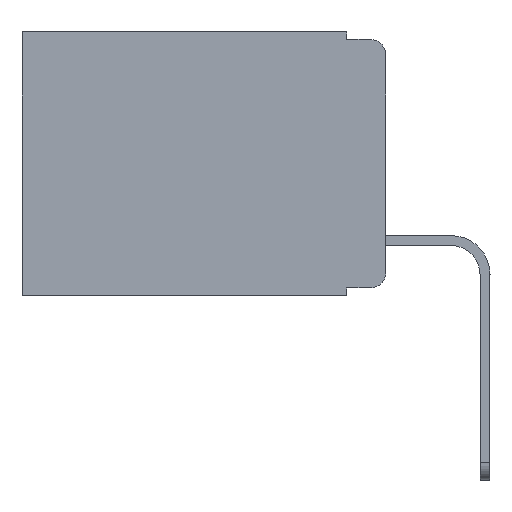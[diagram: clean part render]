
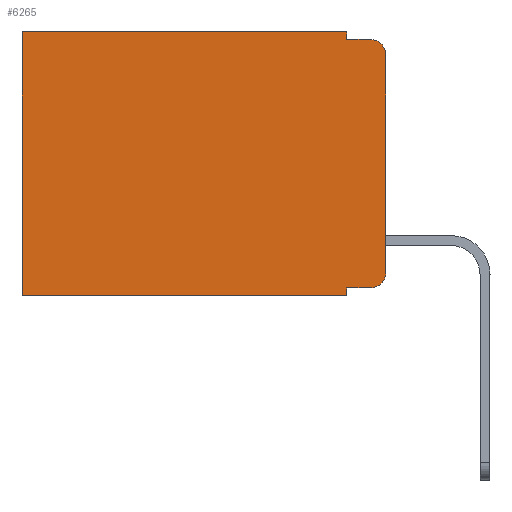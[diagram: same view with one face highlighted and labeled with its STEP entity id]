
A CAD part, left-side view. The second image highlights one B-rep face of the part: STEP entity #6265.
In plain terms, the highlighted planar face has unit normal (-1, 0, 0).
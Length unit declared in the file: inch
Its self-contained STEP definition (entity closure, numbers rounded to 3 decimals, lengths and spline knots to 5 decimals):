
#1 = DIRECTION ( 'NONE',  ( -1., 0., 0. ) ) ;
#213 = CARTESIAN_POINT ( 'NONE',  ( 0.298, 0.051, 0. ) ) ;
#232 = VECTOR ( 'NONE', #8245, 39.37008 ) ;
#307 = CARTESIAN_POINT ( 'NONE',  ( 0.298, 0., -0.03 ) ) ;
#377 = VERTEX_POINT ( 'NONE', #1714 ) ;
#384 = EDGE_CURVE ( 'NONE', #2175, #824, #5941, .T. ) ;
#426 = VERTEX_POINT ( 'NONE', #5489 ) ;
#437 = CARTESIAN_POINT ( 'NONE',  ( 0.298, 0.051, 0. ) ) ;
#585 = DIRECTION ( 'NONE',  ( 0., 1., 0. ) ) ;
#596 = VERTEX_POINT ( 'NONE', #2726 ) ;
#695 = DIRECTION ( 'NONE',  ( 0., 1., 0. ) ) ;
#696 = EDGE_CURVE ( 'NONE', #6378, #426, #6976, .T. ) ;
#824 = VERTEX_POINT ( 'NONE', #2479 ) ;
#828 = LINE ( 'NONE', #5169, #4038 ) ;
#860 = DIRECTION ( 'NONE',  ( 0., 0., -1. ) ) ;
#998 = ORIENTED_EDGE ( 'NONE', *, *, #384, .F. ) ;
#1063 = VECTOR ( 'NONE', #8640, 39.37008 ) ;
#1069 = VERTEX_POINT ( 'NONE', #3045 ) ;
#1148 = ORIENTED_EDGE ( 'NONE', *, *, #696, .T. ) ;
#1170 = AXIS2_PLACEMENT_3D ( 'NONE', #6147, #3266, #1771 ) ;
#1253 = CARTESIAN_POINT ( 'NONE',  ( 0.298, 0.051, -0.333 ) ) ;
#1263 = AXIS2_PLACEMENT_3D ( 'NONE', #8110, #8171, #3757 ) ;
#1367 = CARTESIAN_POINT ( 'NONE',  ( 0.298, 0.02, -0.313 ) ) ;
#1391 = LINE ( 'NONE', #1253, #1063 ) ;
#1530 = EDGE_CURVE ( 'NONE', #824, #426, #4204, .T. ) ;
#1714 = CARTESIAN_POINT ( 'NONE',  ( 0.298, 0.02, -0.333 ) ) ;
#1771 = DIRECTION ( 'NONE',  ( 0., 0., -1. ) ) ;
#1998 = CIRCLE ( 'NONE', #8696, 0.02 ) ;
#2051 = EDGE_CURVE ( 'NONE', #3313, #1069, #7268, .T. ) ;
#2175 = VERTEX_POINT ( 'NONE', #5159 ) ;
#2244 = VECTOR ( 'NONE', #6953, 39.37008 ) ;
#2419 = FACE_OUTER_BOUND ( 'NONE', #6811, .T. ) ;
#2479 = CARTESIAN_POINT ( 'NONE',  ( 0.298, 0.051, -0.01 ) ) ;
#2575 = VECTOR ( 'NONE', #695, 39.37008 ) ;
#2726 = CARTESIAN_POINT ( 'NONE',  ( 0.298, 0., -0.313 ) ) ;
#3045 = CARTESIAN_POINT ( 'NONE',  ( 0.298, 0.473, -0.343 ) ) ;
#3234 = ORIENTED_EDGE ( 'NONE', *, *, #6607, .T. ) ;
#3266 = DIRECTION ( 'NONE',  ( -1., 0., 0. ) ) ;
#3313 = VERTEX_POINT ( 'NONE', #9242 ) ;
#3611 = DIRECTION ( 'NONE',  ( 0., 0., -1. ) ) ;
#3685 = LINE ( 'NONE', #6192, #8020 ) ;
#3757 = DIRECTION ( 'NONE',  ( 0., 0., -1. ) ) ;
#3792 = ORIENTED_EDGE ( 'NONE', *, *, #1530, .F. ) ;
#4014 = CARTESIAN_POINT ( 'NONE',  ( 0.298, 0.051, -0.333 ) ) ;
#4038 = VECTOR ( 'NONE', #860, 39.37008 ) ;
#4204 = LINE ( 'NONE', #4382, #4769 ) ;
#4310 = CARTESIAN_POINT ( 'NONE',  ( 0.298, 0., -0.343 ) ) ;
#4382 = CARTESIAN_POINT ( 'NONE',  ( 0.298, 0.051, -0.01 ) ) ;
#4627 = LINE ( 'NONE', #5634, #8373 ) ;
#4717 = EDGE_CURVE ( 'NONE', #2175, #7197, #4627, .T. ) ;
#4769 = VECTOR ( 'NONE', #8810, 39.37008 ) ;
#4788 = DIRECTION ( 'NONE',  ( 0., 0., -1. ) ) ;
#4868 = EDGE_CURVE ( 'NONE', #377, #596, #1998, .T. ) ;
#4895 = LINE ( 'NONE', #437, #2244 ) ;
#5151 = ORIENTED_EDGE ( 'NONE', *, *, #5830, .T. ) ;
#5159 = CARTESIAN_POINT ( 'NONE',  ( 0.298, 0.051, 0. ) ) ;
#5169 = CARTESIAN_POINT ( 'NONE',  ( 0.298, 0., 0. ) ) ;
#5489 = CARTESIAN_POINT ( 'NONE',  ( 0.298, 0.02, -0.01 ) ) ;
#5634 = CARTESIAN_POINT ( 'NONE',  ( 0.298, 0., 0. ) ) ;
#5711 = EDGE_CURVE ( 'NONE', #6378, #596, #828, .T. ) ;
#5830 = EDGE_CURVE ( 'NONE', #7197, #1069, #3685, .T. ) ;
#5941 = LINE ( 'NONE', #213, #232 ) ;
#6147 = CARTESIAN_POINT ( 'NONE',  ( 0.298, 0.02, -0.03 ) ) ;
#6192 = CARTESIAN_POINT ( 'NONE',  ( 0.298, 0.473, 0. ) ) ;
#6265 = ADVANCED_FACE ( 'NONE', ( #2419 ), #7360, .F. ) ;
#6378 = VERTEX_POINT ( 'NONE', #307 ) ;
#6502 = VERTEX_POINT ( 'NONE', #4014 ) ;
#6607 = EDGE_CURVE ( 'NONE', #6502, #377, #1391, .T. ) ;
#6628 = ORIENTED_EDGE ( 'NONE', *, *, #4717, .T. ) ;
#6657 = ORIENTED_EDGE ( 'NONE', *, *, #5711, .F. ) ;
#6811 = EDGE_LOOP ( 'NONE', ( #6657, #1148, #3792, #998, #6628, #5151, #7679, #9042, #3234, #7078 ) ) ;
#6953 = DIRECTION ( 'NONE',  ( 0., 0., -1. ) ) ;
#6976 = CIRCLE ( 'NONE', #1170, 0.02 ) ;
#7078 = ORIENTED_EDGE ( 'NONE', *, *, #4868, .T. ) ;
#7197 = VERTEX_POINT ( 'NONE', #8543 ) ;
#7268 = LINE ( 'NONE', #4310, #2575 ) ;
#7360 = PLANE ( 'NONE',  #1263 ) ;
#7679 = ORIENTED_EDGE ( 'NONE', *, *, #2051, .F. ) ;
#8020 = VECTOR ( 'NONE', #4788, 39.37008 ) ;
#8110 = CARTESIAN_POINT ( 'NONE',  ( 0.298, 0., 0. ) ) ;
#8171 = DIRECTION ( 'NONE',  ( 1., 0., 0. ) ) ;
#8245 = DIRECTION ( 'NONE',  ( 0., 0., -1. ) ) ;
#8373 = VECTOR ( 'NONE', #585, 39.37008 ) ;
#8543 = CARTESIAN_POINT ( 'NONE',  ( 0.298, 0.473, 0. ) ) ;
#8640 = DIRECTION ( 'NONE',  ( 0., -1., 0. ) ) ;
#8696 = AXIS2_PLACEMENT_3D ( 'NONE', #1367, #1, #3611 ) ;
#8810 = DIRECTION ( 'NONE',  ( 0., -1., 0. ) ) ;
#9042 = ORIENTED_EDGE ( 'NONE', *, *, #9102, .F. ) ;
#9102 = EDGE_CURVE ( 'NONE', #6502, #3313, #4895, .T. ) ;
#9242 = CARTESIAN_POINT ( 'NONE',  ( 0.298, 0.051, -0.343 ) ) ;
